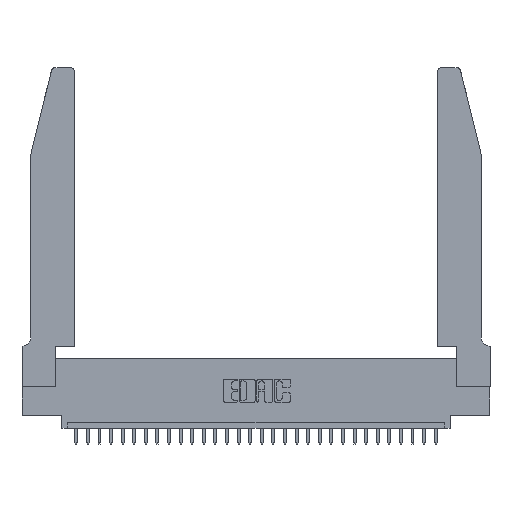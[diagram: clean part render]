
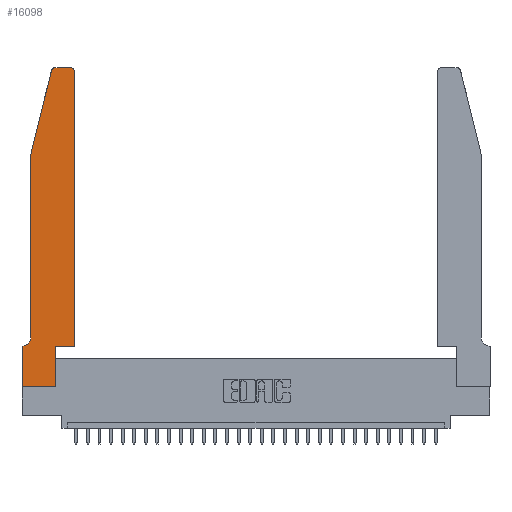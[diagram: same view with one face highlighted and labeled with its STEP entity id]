
A CAD part, top view. The second image highlights one B-rep face of the part: STEP entity #16098.
In plain terms, the highlighted planar face has unit normal (0, 0, 1).
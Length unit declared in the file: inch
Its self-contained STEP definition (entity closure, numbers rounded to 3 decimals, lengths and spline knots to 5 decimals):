
#107 = DIRECTION ( 'NONE',  ( 0., 0., 1. ) ) ;
#145 = CARTESIAN_POINT ( 'NONE',  ( 0.0755, 2., 0.37 ) ) ;
#246 = DIRECTION ( 'NONE',  ( -0.239, -0.971, 0. ) ) ;
#463 = ORIENTED_EDGE ( 'NONE', *, *, #28002, .T. ) ;
#567 = CARTESIAN_POINT ( 'NONE',  ( 0.4205, 2.75, 0.37 ) ) ;
#1043 = CARTESIAN_POINT ( 'NONE',  ( 0.4505, 0.35, 0.37 ) ) ;
#1649 = DIRECTION ( 'NONE',  ( 0., 0., 1. ) ) ;
#2483 = ORIENTED_EDGE ( 'NONE', *, *, #12594, .T. ) ;
#2573 = CARTESIAN_POINT ( 'NONE',  ( 0.2865, 0., 0.37 ) ) ;
#2735 = PLANE ( 'NONE',  #9299 ) ;
#3009 = AXIS2_PLACEMENT_3D ( 'NONE', #22416, #3470, #8347 ) ;
#3402 = VECTOR ( 'NONE', #3779, 39.37008 ) ;
#3470 = DIRECTION ( 'NONE',  ( 0., 0., -1. ) ) ;
#3779 = DIRECTION ( 'NONE',  ( 1., 0., 0. ) ) ;
#3793 = EDGE_LOOP ( 'NONE', ( #463, #18463, #22705, #12297, #5296, #9451, #22529, #14874, #4047, #2483, #13910, #26495 ) ) ;
#3974 = CARTESIAN_POINT ( 'NONE',  ( 0., 0., 0.37 ) ) ;
#4047 = ORIENTED_EDGE ( 'NONE', *, *, #9295, .T. ) ;
#4487 = CARTESIAN_POINT ( 'NONE',  ( 0.0755, 2., 0.37 ) ) ;
#4574 = EDGE_CURVE ( 'NONE', #12167, #5910, #28727, .T. ) ;
#5296 = ORIENTED_EDGE ( 'NONE', *, *, #24898, .T. ) ;
#5380 = CARTESIAN_POINT ( 'NONE',  ( 0.0755, 0.35, 0.37 ) ) ;
#5753 = LINE ( 'NONE', #17040, #29637 ) ;
#5910 = VERTEX_POINT ( 'NONE', #23272 ) ;
#7191 = DIRECTION ( 'NONE',  ( 1., 0., 0. ) ) ;
#7640 = LINE ( 'NONE', #145, #23095 ) ;
#7737 = CARTESIAN_POINT ( 'NONE',  ( 0.0755, 2., 0.37 ) ) ;
#8347 = DIRECTION ( 'NONE',  ( -1., 0., 0. ) ) ;
#8625 = CARTESIAN_POINT ( 'NONE',  ( 0.4505, 0.35, 0.37 ) ) ;
#8864 = DIRECTION ( 'NONE',  ( 0., -1., 0. ) ) ;
#9262 = AXIS2_PLACEMENT_3D ( 'NONE', #22967, #1649, #20366 ) ;
#9295 = EDGE_CURVE ( 'NONE', #16820, #15892, #5753, .T. ) ;
#9299 = AXIS2_PLACEMENT_3D ( 'NONE', #19104, #107, #7191 ) ;
#9436 = CIRCLE ( 'NONE', #3009, 0.07 ) ;
#9451 = ORIENTED_EDGE ( 'NONE', *, *, #18950, .T. ) ;
#9991 = LINE ( 'NONE', #8625, #21406 ) ;
#10451 = VERTEX_POINT ( 'NONE', #21948 ) ;
#10725 = VERTEX_POINT ( 'NONE', #27857 ) ;
#11442 = LINE ( 'NONE', #15003, #13259 ) ;
#11644 = VERTEX_POINT ( 'NONE', #26651 ) ;
#12167 = VERTEX_POINT ( 'NONE', #7737 ) ;
#12185 = LINE ( 'NONE', #3974, #3402 ) ;
#12244 = DIRECTION ( 'NONE',  ( 0., 1., 0. ) ) ;
#12297 = ORIENTED_EDGE ( 'NONE', *, *, #4574, .T. ) ;
#12594 = EDGE_CURVE ( 'NONE', #15892, #23525, #9991, .T. ) ;
#12991 = VECTOR ( 'NONE', #29516, 39.37008 ) ;
#13259 = VECTOR ( 'NONE', #17553, 39.37008 ) ;
#13910 = ORIENTED_EDGE ( 'NONE', *, *, #26666, .T. ) ;
#14085 = LINE ( 'NONE', #1043, #12991 ) ;
#14542 = EDGE_CURVE ( 'NONE', #11644, #14945, #26787, .T. ) ;
#14598 = CIRCLE ( 'NONE', #21073, 0.03 ) ;
#14713 = VERTEX_POINT ( 'NONE', #18628 ) ;
#14874 = ORIENTED_EDGE ( 'NONE', *, *, #27582, .T. ) ;
#14945 = VERTEX_POINT ( 'NONE', #567 ) ;
#14956 = EDGE_CURVE ( 'NONE', #10451, #12167, #7640, .T. ) ;
#14959 = CARTESIAN_POINT ( 'NONE',  ( 0.4505, 0.35, 0.37 ) ) ;
#15003 = CARTESIAN_POINT ( 'NONE',  ( 0.2605, 2.75, 0.37 ) ) ;
#15132 = EDGE_CURVE ( 'NONE', #26745, #10451, #14598, .T. ) ;
#15835 = VECTOR ( 'NONE', #8864, 39.37008 ) ;
#15892 = VERTEX_POINT ( 'NONE', #27656 ) ;
#16098 = ADVANCED_FACE ( 'NONE', ( #27347 ), #2735, .T. ) ;
#16820 = VERTEX_POINT ( 'NONE', #2573 ) ;
#17040 = CARTESIAN_POINT ( 'NONE',  ( 0.2865, 0.35, 0.37 ) ) ;
#17480 = CARTESIAN_POINT ( 'NONE',  ( 0.284, 2.72, 0.37 ) ) ;
#17491 = VERTEX_POINT ( 'NONE', #26855 ) ;
#17553 = DIRECTION ( 'NONE',  ( -1., 0., 0. ) ) ;
#18463 = ORIENTED_EDGE ( 'NONE', *, *, #15132, .T. ) ;
#18628 = CARTESIAN_POINT ( 'NONE',  ( 0., 0., 0.37 ) ) ;
#18950 = EDGE_CURVE ( 'NONE', #10725, #17491, #27938, .T. ) ;
#19104 = CARTESIAN_POINT ( 'NONE',  ( 0., 0.35, 0.37 ) ) ;
#19959 = DIRECTION ( 'NONE',  ( 1., 0., 0. ) ) ;
#20366 = DIRECTION ( 'NONE',  ( 1., 0., 0. ) ) ;
#21019 = EDGE_CURVE ( 'NONE', #17491, #14713, #25225, .T. ) ;
#21073 = AXIS2_PLACEMENT_3D ( 'NONE', #17480, #22036, #19959 ) ;
#21406 = VECTOR ( 'NONE', #30004, 39.37008 ) ;
#21667 = VECTOR ( 'NONE', #29171, 39.37008 ) ;
#21772 = DIRECTION ( 'NONE',  ( 0., -1., 0. ) ) ;
#21948 = CARTESIAN_POINT ( 'NONE',  ( 0.25487, 2.72718, 0.37 ) ) ;
#22036 = DIRECTION ( 'NONE',  ( 0., 0., 1. ) ) ;
#22416 = CARTESIAN_POINT ( 'NONE',  ( 0.0055, 0.42, 0.37 ) ) ;
#22529 = ORIENTED_EDGE ( 'NONE', *, *, #21019, .T. ) ;
#22705 = ORIENTED_EDGE ( 'NONE', *, *, #14956, .T. ) ;
#22967 = CARTESIAN_POINT ( 'NONE',  ( 0.4205, 2.72, 0.37 ) ) ;
#23095 = VECTOR ( 'NONE', #246, 39.37008 ) ;
#23272 = CARTESIAN_POINT ( 'NONE',  ( 0.0755, 0.42, 0.37 ) ) ;
#23525 = VERTEX_POINT ( 'NONE', #14959 ) ;
#24860 = VECTOR ( 'NONE', #21772, 39.37008 ) ;
#24898 = EDGE_CURVE ( 'NONE', #5910, #10725, #9436, .T. ) ;
#25225 = LINE ( 'NONE', #28784, #24860 ) ;
#26495 = ORIENTED_EDGE ( 'NONE', *, *, #14542, .T. ) ;
#26651 = CARTESIAN_POINT ( 'NONE',  ( 0.4505, 2.72, 0.37 ) ) ;
#26666 = EDGE_CURVE ( 'NONE', #23525, #11644, #14085, .T. ) ;
#26745 = VERTEX_POINT ( 'NONE', #29214 ) ;
#26787 = CIRCLE ( 'NONE', #9262, 0.03 ) ;
#26855 = CARTESIAN_POINT ( 'NONE',  ( 0., 0.35, 0.37 ) ) ;
#27347 = FACE_OUTER_BOUND ( 'NONE', #3793, .T. ) ;
#27582 = EDGE_CURVE ( 'NONE', #14713, #16820, #12185, .T. ) ;
#27656 = CARTESIAN_POINT ( 'NONE',  ( 0.2865, 0.35, 0.37 ) ) ;
#27857 = CARTESIAN_POINT ( 'NONE',  ( 0.0055, 0.35, 0.37 ) ) ;
#27938 = LINE ( 'NONE', #5380, #21667 ) ;
#28002 = EDGE_CURVE ( 'NONE', #14945, #26745, #11442, .T. ) ;
#28727 = LINE ( 'NONE', #4487, #15835 ) ;
#28784 = CARTESIAN_POINT ( 'NONE',  ( 0., 0., 0.37 ) ) ;
#29171 = DIRECTION ( 'NONE',  ( -1., 0., 0. ) ) ;
#29214 = CARTESIAN_POINT ( 'NONE',  ( 0.284, 2.75, 0.37 ) ) ;
#29516 = DIRECTION ( 'NONE',  ( 0., 1., 0. ) ) ;
#29637 = VECTOR ( 'NONE', #12244, 39.37008 ) ;
#30004 = DIRECTION ( 'NONE',  ( 1., 0., 0. ) ) ;
